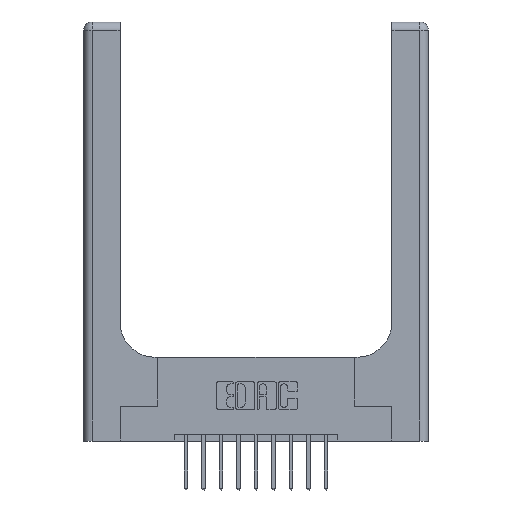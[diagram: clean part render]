
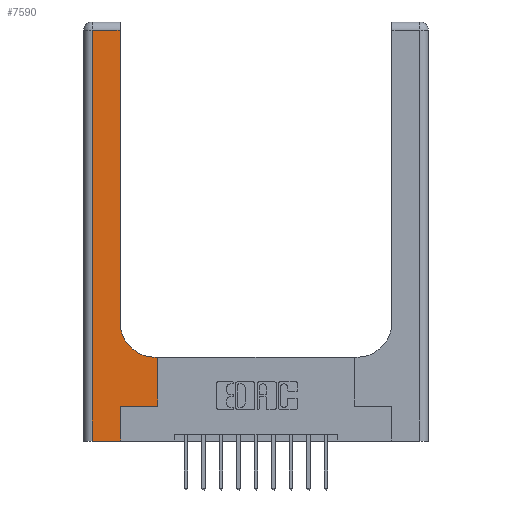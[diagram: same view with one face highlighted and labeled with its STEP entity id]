
A CAD part, top view. The second image highlights one B-rep face of the part: STEP entity #7590.
In plain terms, the highlighted planar face has unit normal (0, 0, 1).
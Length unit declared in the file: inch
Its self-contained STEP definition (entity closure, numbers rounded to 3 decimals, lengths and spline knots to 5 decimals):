
#86 = EDGE_CURVE ( 'NONE', #6759, #14686, #3287, .T. ) ;
#242 = DIRECTION ( 'NONE',  ( 0., 1., 0. ) ) ;
#446 = DIRECTION ( 'NONE',  ( 0., 1., 0. ) ) ;
#523 = EDGE_LOOP ( 'NONE', ( #6194, #10605, #4352, #4405, #4860, #4080, #6369, #4840, #6361 ) ) ;
#655 = LINE ( 'NONE', #4200, #2925 ) ;
#658 = EDGE_CURVE ( 'NONE', #14686, #6022, #6372, .T. ) ;
#787 = VECTOR ( 'NONE', #1996, 39.37008 ) ;
#1996 = DIRECTION ( 'NONE',  ( -1., 0., 0. ) ) ;
#2770 = CARTESIAN_POINT ( 'NONE',  ( 0.26, 3., 0.37 ) ) ;
#2925 = VECTOR ( 'NONE', #11452, 39.37008 ) ;
#2929 = VERTEX_POINT ( 'NONE', #10273 ) ;
#3018 = EDGE_CURVE ( 'NONE', #7844, #10816, #11493, .T. ) ;
#3149 = CARTESIAN_POINT ( 'NONE',  ( 0.265, 0., 0.37 ) ) ;
#3196 = VECTOR ( 'NONE', #5656, 39.37008 ) ;
#3287 = LINE ( 'NONE', #8189, #13513 ) ;
#3863 = DIRECTION ( 'NONE',  ( -1., 0., 0. ) ) ;
#4080 = ORIENTED_EDGE ( 'NONE', *, *, #8877, .T. ) ;
#4087 = CARTESIAN_POINT ( 'NONE',  ( 0.528, 0.25, 0.37 ) ) ;
#4200 = CARTESIAN_POINT ( 'NONE',  ( 0.265, 0.25, 0.37 ) ) ;
#4215 = DIRECTION ( 'NONE',  ( -1., 0., 0. ) ) ;
#4321 = EDGE_CURVE ( 'NONE', #10816, #9833, #5796, .T. ) ;
#4352 = ORIENTED_EDGE ( 'NONE', *, *, #9076, .T. ) ;
#4405 = ORIENTED_EDGE ( 'NONE', *, *, #86, .T. ) ;
#4840 = ORIENTED_EDGE ( 'NONE', *, *, #4321, .T. ) ;
#4860 = ORIENTED_EDGE ( 'NONE', *, *, #658, .T. ) ;
#5080 = PLANE ( 'NONE',  #12164 ) ;
#5508 = DIRECTION ( 'NONE',  ( 1., 0., 0. ) ) ;
#5656 = DIRECTION ( 'NONE',  ( 0., -1., 0. ) ) ;
#5749 = DIRECTION ( 'NONE',  ( 0., 0., -1. ) ) ;
#5796 = LINE ( 'NONE', #10695, #787 ) ;
#6020 = EDGE_CURVE ( 'NONE', #2929, #15949, #9707, .T. ) ;
#6022 = VERTEX_POINT ( 'NONE', #14062 ) ;
#6194 = ORIENTED_EDGE ( 'NONE', *, *, #8319, .T. ) ;
#6361 = ORIENTED_EDGE ( 'NONE', *, *, #11067, .T. ) ;
#6369 = ORIENTED_EDGE ( 'NONE', *, *, #3018, .T. ) ;
#6372 = LINE ( 'NONE', #7588, #13754 ) ;
#6748 = CARTESIAN_POINT ( 'NONE',  ( 0.26, 0.85, 0.37 ) ) ;
#6759 = VERTEX_POINT ( 'NONE', #9744 ) ;
#7588 = CARTESIAN_POINT ( 'NONE',  ( 0.265, 0., 0.37 ) ) ;
#7590 = ADVANCED_FACE ( 'NONE', ( #11199 ), #5080, .F. ) ;
#7844 = VERTEX_POINT ( 'NONE', #9960 ) ;
#8189 = CARTESIAN_POINT ( 'NONE',  ( 0., 0., 0.37 ) ) ;
#8296 = AXIS2_PLACEMENT_3D ( 'NONE', #9521, #5749, #5508 ) ;
#8319 = EDGE_CURVE ( 'NONE', #10575, #2929, #10013, .T. ) ;
#8877 = EDGE_CURVE ( 'NONE', #6022, #7844, #655, .T. ) ;
#9076 = EDGE_CURVE ( 'NONE', #15949, #6759, #9514, .T. ) ;
#9514 = LINE ( 'NONE', #12107, #3196 ) ;
#9521 = CARTESIAN_POINT ( 'NONE',  ( 0.51, 0.85, 0.37 ) ) ;
#9707 = LINE ( 'NONE', #10007, #14701 ) ;
#9744 = CARTESIAN_POINT ( 'NONE',  ( 0.06, 0., 0.37 ) ) ;
#9833 = VERTEX_POINT ( 'NONE', #15762 ) ;
#9960 = CARTESIAN_POINT ( 'NONE',  ( 0.528, 0.25, 0.37 ) ) ;
#10007 = CARTESIAN_POINT ( 'NONE',  ( 0., 2.94, 0.37 ) ) ;
#10013 = LINE ( 'NONE', #2770, #15793 ) ;
#10273 = CARTESIAN_POINT ( 'NONE',  ( 0.26, 2.94, 0.37 ) ) ;
#10575 = VERTEX_POINT ( 'NONE', #6748 ) ;
#10605 = ORIENTED_EDGE ( 'NONE', *, *, #6020, .T. ) ;
#10695 = CARTESIAN_POINT ( 'NONE',  ( 0.26, 0.6, 0.37 ) ) ;
#10816 = VERTEX_POINT ( 'NONE', #12459 ) ;
#11067 = EDGE_CURVE ( 'NONE', #9833, #10575, #13956, .T. ) ;
#11199 = FACE_OUTER_BOUND ( 'NONE', #523, .T. ) ;
#11452 = DIRECTION ( 'NONE',  ( 1., 0., 0. ) ) ;
#11493 = LINE ( 'NONE', #4087, #13467 ) ;
#12107 = CARTESIAN_POINT ( 'NONE',  ( 0.06, 3., 0.37 ) ) ;
#12164 = AXIS2_PLACEMENT_3D ( 'NONE', #14908, #12558, #3863 ) ;
#12459 = CARTESIAN_POINT ( 'NONE',  ( 0.528, 0.6, 0.37 ) ) ;
#12558 = DIRECTION ( 'NONE',  ( 0., 0., -1. ) ) ;
#13101 = DIRECTION ( 'NONE',  ( 1., 0., 0. ) ) ;
#13467 = VECTOR ( 'NONE', #446, 39.37008 ) ;
#13513 = VECTOR ( 'NONE', #13101, 39.37008 ) ;
#13754 = VECTOR ( 'NONE', #242, 39.37008 ) ;
#13956 = CIRCLE ( 'NONE', #8296, 0.25 ) ;
#14062 = CARTESIAN_POINT ( 'NONE',  ( 0.265, 0.25, 0.37 ) ) ;
#14686 = VERTEX_POINT ( 'NONE', #3149 ) ;
#14701 = VECTOR ( 'NONE', #4215, 39.37008 ) ;
#14872 = DIRECTION ( 'NONE',  ( 0., 1., 0. ) ) ;
#14908 = CARTESIAN_POINT ( 'NONE',  ( 0., 3., 0.37 ) ) ;
#15716 = CARTESIAN_POINT ( 'NONE',  ( 0.06, 2.94, 0.37 ) ) ;
#15762 = CARTESIAN_POINT ( 'NONE',  ( 0.51, 0.6, 0.37 ) ) ;
#15793 = VECTOR ( 'NONE', #14872, 39.37008 ) ;
#15949 = VERTEX_POINT ( 'NONE', #15716 ) ;
